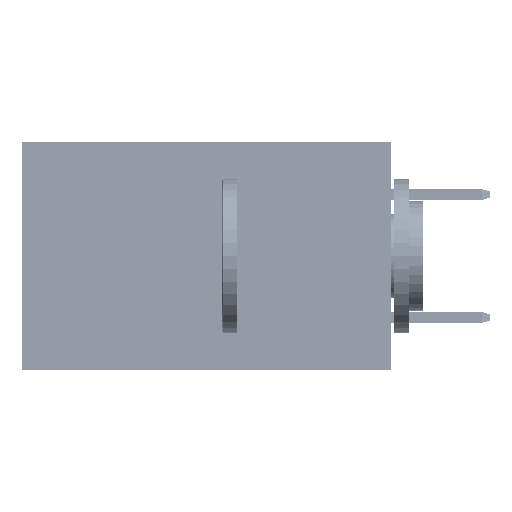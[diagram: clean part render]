
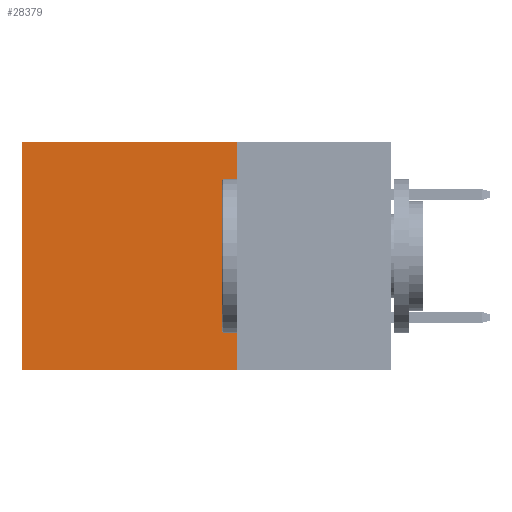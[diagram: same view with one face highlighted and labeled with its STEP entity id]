
A CAD part, left-side view. The second image highlights one B-rep face of the part: STEP entity #28379.
In plain terms, the highlighted planar face has unit normal (-1, 0, 0).
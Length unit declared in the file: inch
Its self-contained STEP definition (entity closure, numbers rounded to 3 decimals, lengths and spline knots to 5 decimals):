
#1088 = VECTOR ( 'NONE', #26145, 39.37008 ) ;
#1979 = VERTEX_POINT ( 'NONE', #29100 ) ;
#2330 = EDGE_CURVE ( 'NONE', #10505, #1979, #13904, .T. ) ;
#4374 = CARTESIAN_POINT ( 'NONE',  ( 0.2875, 0.25, -0.37 ) ) ;
#7024 = CARTESIAN_POINT ( 'NONE',  ( 0.2875, 0.25, -0.37 ) ) ;
#10255 = CARTESIAN_POINT ( 'NONE',  ( 0.2875, 0.6, 0. ) ) ;
#10505 = VERTEX_POINT ( 'NONE', #10627 ) ;
#10627 = CARTESIAN_POINT ( 'NONE',  ( 0.2875, 0.6, 0. ) ) ;
#12511 = DIRECTION ( 'NONE',  ( 0., 0., -1. ) ) ;
#12548 = VERTEX_POINT ( 'NONE', #45669 ) ;
#13167 = EDGE_CURVE ( 'NONE', #21540, #1979, #29719, .T. ) ;
#13426 = ORIENTED_EDGE ( 'NONE', *, *, #2330, .T. ) ;
#13904 = LINE ( 'NONE', #10255, #15071 ) ;
#15071 = VECTOR ( 'NONE', #28804, 39.37008 ) ;
#15454 = LINE ( 'NONE', #38918, #37253 ) ;
#17502 = AXIS2_PLACEMENT_3D ( 'NONE', #39034, #28118, #45845 ) ;
#18722 = LINE ( 'NONE', #26929, #46716 ) ;
#21540 = VERTEX_POINT ( 'NONE', #7024 ) ;
#24122 = ORIENTED_EDGE ( 'NONE', *, *, #13167, .F. ) ;
#26145 = DIRECTION ( 'NONE',  ( 0., 1., 0. ) ) ;
#26929 = CARTESIAN_POINT ( 'NONE',  ( 0.2875, 0.25, 0. ) ) ;
#28009 = DIRECTION ( 'NONE',  ( 0., 1., 0. ) ) ;
#28118 = DIRECTION ( 'NONE',  ( 1., 0., 0. ) ) ;
#28379 = ADVANCED_FACE ( 'NONE', ( #32339 ), #46159, .F. ) ;
#28804 = DIRECTION ( 'NONE',  ( 0., 0., -1. ) ) ;
#29100 = CARTESIAN_POINT ( 'NONE',  ( 0.2875, 0.6, -0.37 ) ) ;
#29719 = LINE ( 'NONE', #4374, #1088 ) ;
#31550 = EDGE_CURVE ( 'NONE', #12548, #10505, #15454, .T. ) ;
#31863 = ORIENTED_EDGE ( 'NONE', *, *, #33372, .F. ) ;
#32339 = FACE_OUTER_BOUND ( 'NONE', #42317, .T. ) ;
#33372 = EDGE_CURVE ( 'NONE', #12548, #21540, #18722, .T. ) ;
#35830 = ORIENTED_EDGE ( 'NONE', *, *, #31550, .T. ) ;
#37253 = VECTOR ( 'NONE', #28009, 39.37008 ) ;
#38918 = CARTESIAN_POINT ( 'NONE',  ( 0.2875, 0.25, 0. ) ) ;
#39034 = CARTESIAN_POINT ( 'NONE',  ( 0.2875, 0.25, 0. ) ) ;
#42317 = EDGE_LOOP ( 'NONE', ( #13426, #24122, #31863, #35830 ) ) ;
#45669 = CARTESIAN_POINT ( 'NONE',  ( 0.2875, 0.25, 0. ) ) ;
#45845 = DIRECTION ( 'NONE',  ( 0., 0., -1. ) ) ;
#46159 = PLANE ( 'NONE',  #17502 ) ;
#46716 = VECTOR ( 'NONE', #12511, 39.37008 ) ;
